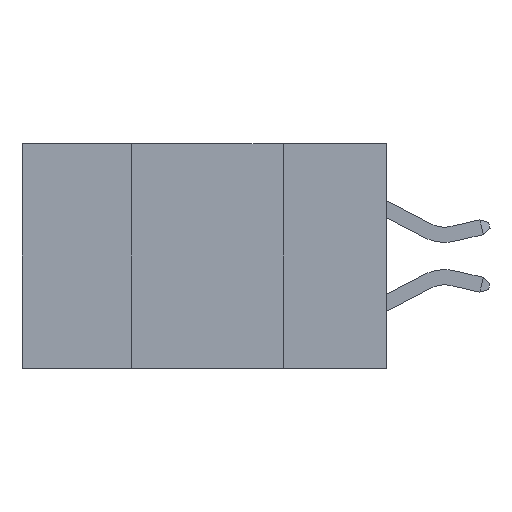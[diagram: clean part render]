
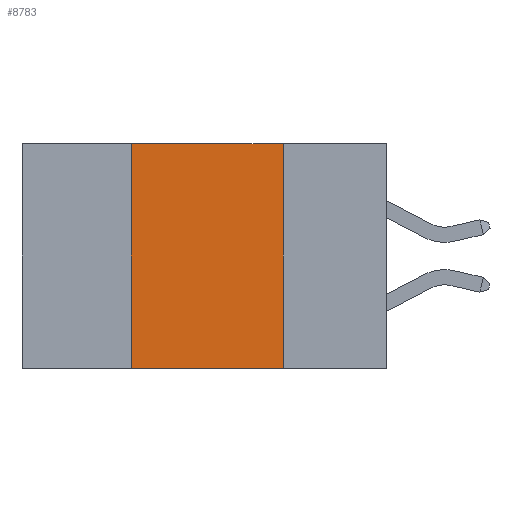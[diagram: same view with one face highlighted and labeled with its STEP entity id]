
A CAD part, left-side view. The second image highlights one B-rep face of the part: STEP entity #8783.
In plain terms, the highlighted planar face has unit normal (-1, 0, 0).
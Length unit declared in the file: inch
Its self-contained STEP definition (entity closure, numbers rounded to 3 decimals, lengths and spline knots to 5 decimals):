
#699 = VECTOR ( 'NONE', #1567, 39.37008 ) ;
#701 = DIRECTION ( 'NONE',  ( 0., 0., 1. ) ) ;
#824 = CARTESIAN_POINT ( 'NONE',  ( 0., 0.17, 0. ) ) ;
#1326 = VERTEX_POINT ( 'NONE', #8781 ) ;
#1383 = EDGE_CURVE ( 'NONE', #8173, #8389, #11744, .T. ) ;
#1567 = DIRECTION ( 'NONE',  ( 0., -1., 0. ) ) ;
#1846 = CARTESIAN_POINT ( 'NONE',  ( 0., 0.17, 0. ) ) ;
#3248 = CARTESIAN_POINT ( 'NONE',  ( 0., 0.6, -0.37 ) ) ;
#3402 = LINE ( 'NONE', #1846, #9789 ) ;
#4189 = EDGE_CURVE ( 'NONE', #1326, #13093, #11647, .T. ) ;
#4719 = CARTESIAN_POINT ( 'NONE',  ( 0., 0.6, 0. ) ) ;
#4720 = CARTESIAN_POINT ( 'NONE',  ( 0., 0.42, -0.37 ) ) ;
#4966 = ORIENTED_EDGE ( 'NONE', *, *, #4189, .F. ) ;
#5063 = EDGE_LOOP ( 'NONE', ( #7479, #4966, #7328, #5421 ) ) ;
#5421 = ORIENTED_EDGE ( 'NONE', *, *, #1383, .T. ) ;
#7292 = PLANE ( 'NONE',  #7389 ) ;
#7328 = ORIENTED_EDGE ( 'NONE', *, *, #16326, .F. ) ;
#7389 = AXIS2_PLACEMENT_3D ( 'NONE', #8602, #16596, #8663 ) ;
#7479 = ORIENTED_EDGE ( 'NONE', *, *, #17352, .F. ) ;
#8160 = FACE_OUTER_BOUND ( 'NONE', #5063, .T. ) ;
#8173 = VERTEX_POINT ( 'NONE', #4720 ) ;
#8389 = VERTEX_POINT ( 'NONE', #10531 ) ;
#8602 = CARTESIAN_POINT ( 'NONE',  ( 0., 0.6, 0. ) ) ;
#8663 = DIRECTION ( 'NONE',  ( 0., 0., -1. ) ) ;
#8735 = DIRECTION ( 'NONE',  ( 0., -1., 0. ) ) ;
#8781 = CARTESIAN_POINT ( 'NONE',  ( 0., 0.42, 0. ) ) ;
#8783 = ADVANCED_FACE ( 'NONE', ( #8160 ), #7292, .F. ) ;
#9789 = VECTOR ( 'NONE', #16686, 39.37008 ) ;
#10053 = VECTOR ( 'NONE', #701, 39.37008 ) ;
#10531 = CARTESIAN_POINT ( 'NONE',  ( 0., 0.17, -0.37 ) ) ;
#11647 = LINE ( 'NONE', #4719, #699 ) ;
#11744 = LINE ( 'NONE', #3248, #14786 ) ;
#13093 = VERTEX_POINT ( 'NONE', #824 ) ;
#14202 = CARTESIAN_POINT ( 'NONE',  ( 0., 0.42, 0. ) ) ;
#14786 = VECTOR ( 'NONE', #8735, 39.37008 ) ;
#16326 = EDGE_CURVE ( 'NONE', #8173, #1326, #17041, .T. ) ;
#16596 = DIRECTION ( 'NONE',  ( 1., 0., 0. ) ) ;
#16686 = DIRECTION ( 'NONE',  ( 0., 0., -1. ) ) ;
#17041 = LINE ( 'NONE', #14202, #10053 ) ;
#17352 = EDGE_CURVE ( 'NONE', #13093, #8389, #3402, .T. ) ;
